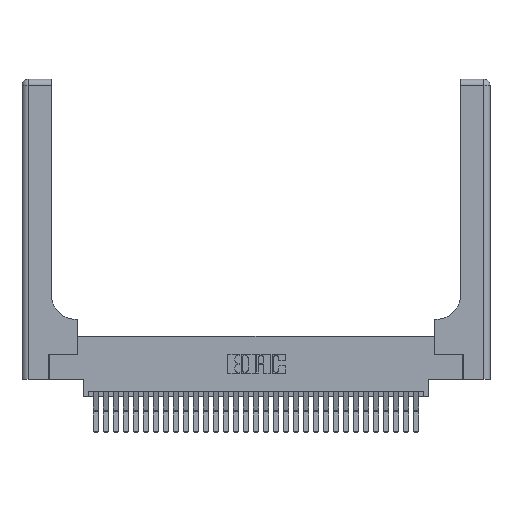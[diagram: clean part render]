
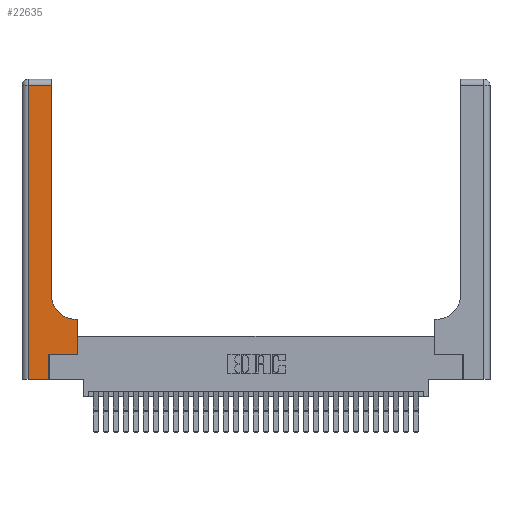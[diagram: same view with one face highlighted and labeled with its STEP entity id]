
A CAD part, top view. The second image highlights one B-rep face of the part: STEP entity #22635.
In plain terms, the highlighted planar face has unit normal (0, 0, 1).
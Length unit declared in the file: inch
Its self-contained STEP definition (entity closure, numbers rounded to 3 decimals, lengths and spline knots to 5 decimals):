
#291 = ORIENTED_EDGE ( 'NONE', *, *, #8777, .T. ) ;
#612 = DIRECTION ( 'NONE',  ( -1., 0., 0. ) ) ;
#935 = ORIENTED_EDGE ( 'NONE', *, *, #32205, .T. ) ;
#1914 = LINE ( 'NONE', #15592, #26254 ) ;
#2087 = VERTEX_POINT ( 'NONE', #7308 ) ;
#3047 = DIRECTION ( 'NONE',  ( 0., 1., 0. ) ) ;
#3055 = CARTESIAN_POINT ( 'NONE',  ( 0., 3., 0.37 ) ) ;
#3162 = LINE ( 'NONE', #13473, #16981 ) ;
#3739 = DIRECTION ( 'NONE',  ( 0., 1., 0. ) ) ;
#4060 = VERTEX_POINT ( 'NONE', #25990 ) ;
#4200 = VERTEX_POINT ( 'NONE', #16274 ) ;
#4252 = VERTEX_POINT ( 'NONE', #6952 ) ;
#4587 = ORIENTED_EDGE ( 'NONE', *, *, #19317, .T. ) ;
#5705 = AXIS2_PLACEMENT_3D ( 'NONE', #3055, #30511, #612 ) ;
#5883 = CARTESIAN_POINT ( 'NONE',  ( 0.2915, 0.6, 0.37 ) ) ;
#5906 = VECTOR ( 'NONE', #10955, 39.37008 ) ;
#6300 = DIRECTION ( 'NONE',  ( 1., 0., 0. ) ) ;
#6366 = DIRECTION ( 'NONE',  ( 1., 0., 0. ) ) ;
#6952 = CARTESIAN_POINT ( 'NONE',  ( 0.2915, 0.85, 0.37 ) ) ;
#7080 = LINE ( 'NONE', #31742, #12213 ) ;
#7308 = CARTESIAN_POINT ( 'NONE',  ( 0.5415, 0.6, 0.37 ) ) ;
#7581 = VERTEX_POINT ( 'NONE', #15831 ) ;
#8381 = EDGE_CURVE ( 'NONE', #26578, #29729, #31178, .T. ) ;
#8607 = DIRECTION ( 'NONE',  ( 0., 0., -1. ) ) ;
#8666 = CARTESIAN_POINT ( 'NONE',  ( 0.269, 0.25, 0.37 ) ) ;
#8685 = DIRECTION ( 'NONE',  ( -1., 0., 0. ) ) ;
#8777 = EDGE_CURVE ( 'NONE', #29874, #4200, #32352, .T. ) ;
#10603 = ORIENTED_EDGE ( 'NONE', *, *, #8381, .T. ) ;
#10955 = DIRECTION ( 'NONE',  ( -1., 0., 0. ) ) ;
#11890 = CIRCLE ( 'NONE', #25995, 0.25 ) ;
#12023 = VECTOR ( 'NONE', #30180, 39.37008 ) ;
#12213 = VECTOR ( 'NONE', #3739, 39.37008 ) ;
#12971 = PLANE ( 'NONE',  #5705 ) ;
#13124 = VECTOR ( 'NONE', #8685, 39.37008 ) ;
#13339 = ORIENTED_EDGE ( 'NONE', *, *, #17230, .T. ) ;
#13473 = CARTESIAN_POINT ( 'NONE',  ( 0.06, 3., 0.37 ) ) ;
#14107 = EDGE_LOOP ( 'NONE', ( #17947, #291, #24417, #935, #31296, #10603, #4587, #14532, #13339 ) ) ;
#14468 = VERTEX_POINT ( 'NONE', #16831 ) ;
#14532 = ORIENTED_EDGE ( 'NONE', *, *, #17502, .T. ) ;
#15231 = CARTESIAN_POINT ( 'NONE',  ( 0.269, 0.25, 0.37 ) ) ;
#15268 = CARTESIAN_POINT ( 'NONE',  ( 0.5585, 0.25, 0.37 ) ) ;
#15592 = CARTESIAN_POINT ( 'NONE',  ( 0.269, 0., 0.37 ) ) ;
#15623 = LINE ( 'NONE', #15268, #27016 ) ;
#15831 = CARTESIAN_POINT ( 'NONE',  ( 0.269, 0., 0.37 ) ) ;
#16176 = CARTESIAN_POINT ( 'NONE',  ( 0., 2.94, 0.37 ) ) ;
#16274 = CARTESIAN_POINT ( 'NONE',  ( 0.06, 2.94, 0.37 ) ) ;
#16831 = CARTESIAN_POINT ( 'NONE',  ( 0.06, 0., 0.37 ) ) ;
#16981 = VECTOR ( 'NONE', #25731, 39.37008 ) ;
#17230 = EDGE_CURVE ( 'NONE', #2087, #4252, #11890, .T. ) ;
#17502 = EDGE_CURVE ( 'NONE', #4060, #2087, #29119, .T. ) ;
#17905 = DIRECTION ( 'NONE',  ( 0., 1., 0. ) ) ;
#17947 = ORIENTED_EDGE ( 'NONE', *, *, #26947, .T. ) ;
#19317 = EDGE_CURVE ( 'NONE', #29729, #4060, #15623, .T. ) ;
#19460 = VECTOR ( 'NONE', #6366, 39.37008 ) ;
#21040 = LINE ( 'NONE', #25222, #12023 ) ;
#21591 = CARTESIAN_POINT ( 'NONE',  ( 0.5415, 0.85, 0.37 ) ) ;
#22381 = CARTESIAN_POINT ( 'NONE',  ( 0.5585, 0.25, 0.37 ) ) ;
#22635 = ADVANCED_FACE ( 'NONE', ( #30859 ), #12971, .F. ) ;
#22955 = CARTESIAN_POINT ( 'NONE',  ( 0.2915, 2.94, 0.37 ) ) ;
#24417 = ORIENTED_EDGE ( 'NONE', *, *, #28069, .T. ) ;
#25222 = CARTESIAN_POINT ( 'NONE',  ( 0., 0., 0.37 ) ) ;
#25731 = DIRECTION ( 'NONE',  ( 0., -1., 0. ) ) ;
#25990 = CARTESIAN_POINT ( 'NONE',  ( 0.5585, 0.6, 0.37 ) ) ;
#25995 = AXIS2_PLACEMENT_3D ( 'NONE', #21591, #8607, #6300 ) ;
#26254 = VECTOR ( 'NONE', #17905, 39.37008 ) ;
#26578 = VERTEX_POINT ( 'NONE', #15231 ) ;
#26947 = EDGE_CURVE ( 'NONE', #4252, #29874, #7080, .T. ) ;
#27016 = VECTOR ( 'NONE', #3047, 39.37008 ) ;
#27432 = EDGE_CURVE ( 'NONE', #7581, #26578, #1914, .T. ) ;
#28069 = EDGE_CURVE ( 'NONE', #4200, #14468, #3162, .T. ) ;
#29119 = LINE ( 'NONE', #5883, #5906 ) ;
#29729 = VERTEX_POINT ( 'NONE', #22381 ) ;
#29874 = VERTEX_POINT ( 'NONE', #22955 ) ;
#30180 = DIRECTION ( 'NONE',  ( 1., 0., 0. ) ) ;
#30511 = DIRECTION ( 'NONE',  ( 0., 0., -1. ) ) ;
#30859 = FACE_OUTER_BOUND ( 'NONE', #14107, .T. ) ;
#31178 = LINE ( 'NONE', #8666, #19460 ) ;
#31296 = ORIENTED_EDGE ( 'NONE', *, *, #27432, .T. ) ;
#31742 = CARTESIAN_POINT ( 'NONE',  ( 0.2915, 3., 0.37 ) ) ;
#32205 = EDGE_CURVE ( 'NONE', #14468, #7581, #21040, .T. ) ;
#32352 = LINE ( 'NONE', #16176, #13124 ) ;
